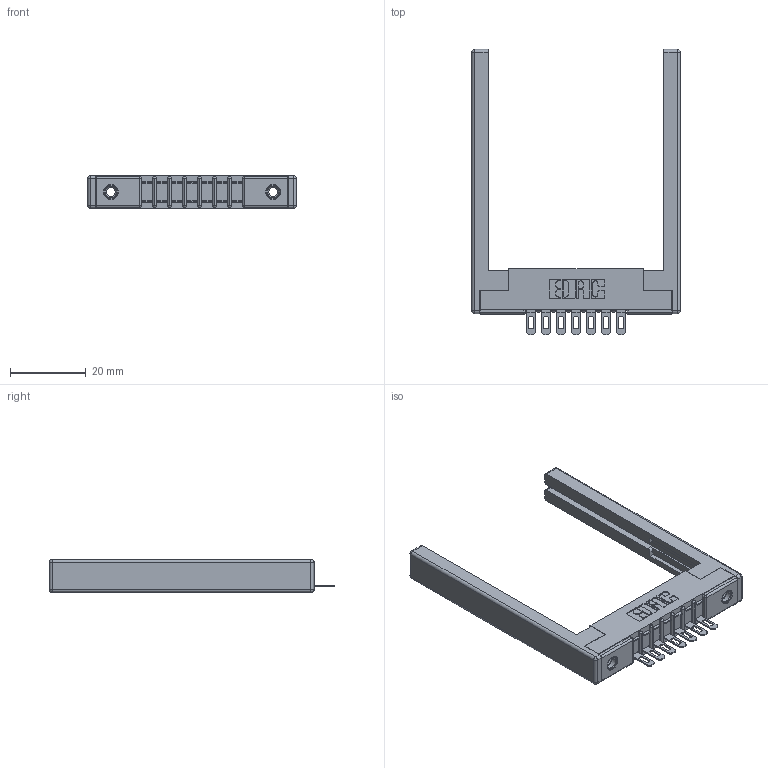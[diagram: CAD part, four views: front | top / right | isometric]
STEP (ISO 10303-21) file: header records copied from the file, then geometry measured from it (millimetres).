
FILE_DESCRIPTION (( 'STEP AP203' ), '1' );
FILE_NAME ('307-007-401-168.STEP', '2020-09-25T02:12:56', ( '' ), ( '' ), 'SwSTEP 2.0', 'SolidWorks 2020', '' );
FILE_SCHEMA (( 'CONFIG_CONTROL_DESIGN' ));
Length unit declared in the file: inch
Products named in the file (5): 345-250-001_345-250-001-102; 307-290-002_501; 307-007-401-168; 307 Part_.156 Dia Mounting Holes; 307-220-068
Assembly tree (12 placements, depth 2):
  307-007-401-168
    307 Part_.156 Dia Mounting Holes
    307-290-002_501  x7
    307-220-068  x2
    345-250-001_345-250-001-102  x2
Bounding box: 55.17 x 75.39 x 8.71 mm (x, y, z)
Volume: 8199.2 mm3; surface area: 9854.9 mm2
Topology: 12 solids, 12 shells, 812 faces, 2379 edges, 1542 vertices
Faces by surface type: plane 466, cylinder 306, sphere 24, cone 12, torus 4
Entity records: 13869 total; most frequent: CARTESIAN_POINT 2297, ORIENTED_EDGE 2276, DIRECTION 2270, EDGE_CURVE 1138, VECTOR 848, LINE 848, VERTEX_POINT 738, AXIS2_PLACEMENT_3D 711
